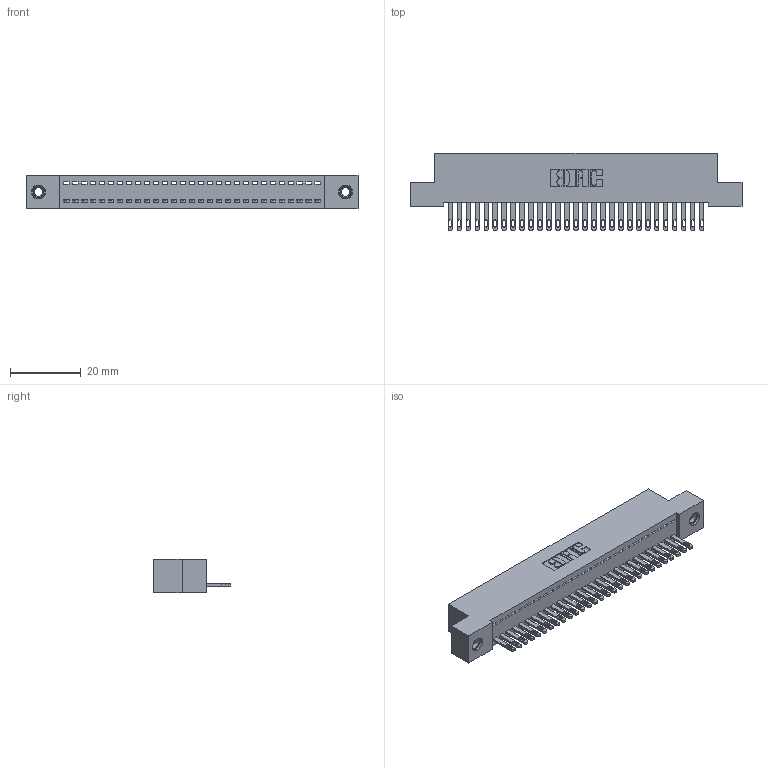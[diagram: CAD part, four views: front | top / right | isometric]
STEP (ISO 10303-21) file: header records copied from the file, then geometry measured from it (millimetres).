
FILE_DESCRIPTION (( 'STEP AP203' ), '1' );
FILE_NAME ('342-029-500-107.STEP', '2018-08-11T14:40:39', ( '' ), ( '' ), 'SwSTEP 2.0', 'SolidWorks 2016', '' );
FILE_SCHEMA (( 'CONFIG_CONTROL_DESIGN' ));
Length unit declared in the file: inch
Products named in the file (4): 342 Part_TI; 345-292-001_345-293-100; 345-250-001_345-250-005-103; 342-029-500-107
Assembly tree (32 placements, depth 2):
  342-029-500-107
    342 Part_TI
    345-292-001_345-293-100  x29
    345-250-001_345-250-005-103  x2
Bounding box: 93.98 x 21.85 x 9.4 mm (x, y, z)
Volume: 8197.5 mm3; surface area: 11884.3 mm2
Topology: 32 solids, 32 shells, 1736 faces, 5307 edges, 3530 vertices
Faces by surface type: plane 1142, cylinder 578, cone 12, torus 4
Entity records: 20394 total; most frequent: CARTESIAN_POINT 3500, ORIENTED_EDGE 3458, DIRECTION 3013, EDGE_CURVE 1729, VECTOR 1577, LINE 1577, VERTEX_POINT 1148, AXIS2_PLACEMENT_3D 718
